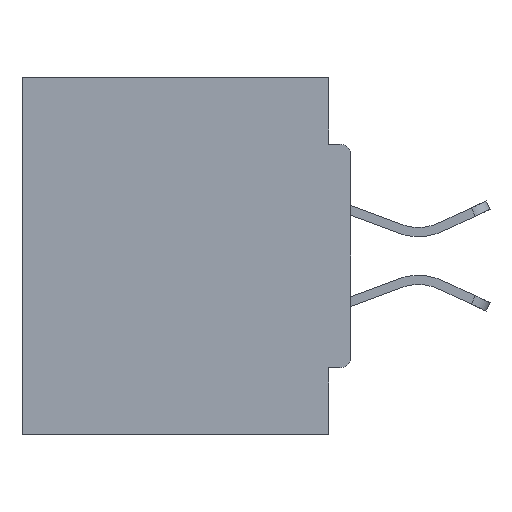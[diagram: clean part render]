
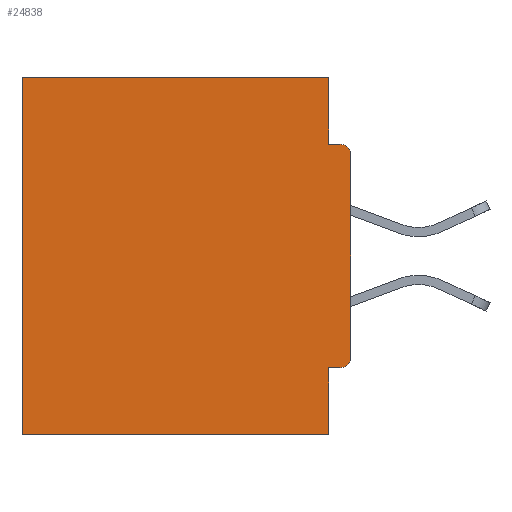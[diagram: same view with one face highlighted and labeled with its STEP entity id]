
A CAD part, left-side view. The second image highlights one B-rep face of the part: STEP entity #24838.
In plain terms, the highlighted planar face has unit normal (-1, 0, 0).
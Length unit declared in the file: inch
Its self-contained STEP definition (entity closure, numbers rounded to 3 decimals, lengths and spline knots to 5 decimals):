
#800 = CARTESIAN_POINT ( 'NONE',  ( 0.298, 0.031, 0. ) ) ;
#1332 = LINE ( 'NONE', #5287, #27914 ) ;
#1962 = LINE ( 'NONE', #23054, #7258 ) ;
#1979 = EDGE_CURVE ( 'NONE', #17527, #6741, #15284, .T. ) ;
#2102 = EDGE_LOOP ( 'NONE', ( #6151, #5456, #30025, #8005, #17587, #11254, #28981, #26179, #26817, #15658 ) ) ;
#2322 = VECTOR ( 'NONE', #16249, 39.37008 ) ;
#2545 = VECTOR ( 'NONE', #28254, 39.37008 ) ;
#3219 = VERTEX_POINT ( 'NONE', #16351 ) ;
#3903 = DIRECTION ( 'NONE',  ( 0., 0., -1. ) ) ;
#4043 = EDGE_CURVE ( 'NONE', #28127, #31841, #24545, .T. ) ;
#4402 = CARTESIAN_POINT ( 'NONE',  ( 0.298, 0., 0. ) ) ;
#5287 = CARTESIAN_POINT ( 'NONE',  ( 0.298, 0., -0.0935 ) ) ;
#5456 = ORIENTED_EDGE ( 'NONE', *, *, #21370, .F. ) ;
#5717 = CARTESIAN_POINT ( 'NONE',  ( 0.298, 0., -0.3915 ) ) ;
#6151 = ORIENTED_EDGE ( 'NONE', *, *, #33785, .T. ) ;
#6346 = AXIS2_PLACEMENT_3D ( 'NONE', #28651, #12652, #20780 ) ;
#6703 = CARTESIAN_POINT ( 'NONE',  ( 0.298, 0.031, -0.5 ) ) ;
#6741 = VERTEX_POINT ( 'NONE', #6703 ) ;
#6881 = DIRECTION ( 'NONE',  ( 0., 0., -1. ) ) ;
#6910 = DIRECTION ( 'NONE',  ( 0., 1., 0. ) ) ;
#7258 = VECTOR ( 'NONE', #28536, 39.37008 ) ;
#7495 = CIRCLE ( 'NONE', #19519, 0.015 ) ;
#7565 = EDGE_CURVE ( 'NONE', #6741, #33610, #25634, .T. ) ;
#8005 = ORIENTED_EDGE ( 'NONE', *, *, #4043, .T. ) ;
#8009 = CARTESIAN_POINT ( 'NONE',  ( 0.298, 0.015, -0.4065 ) ) ;
#9202 = CARTESIAN_POINT ( 'NONE',  ( 0.298, 0.46, 0. ) ) ;
#9961 = CARTESIAN_POINT ( 'NONE',  ( 0.298, 0.031, -0.5 ) ) ;
#9985 = VECTOR ( 'NONE', #30195, 39.37008 ) ;
#10547 = EDGE_CURVE ( 'NONE', #28127, #3219, #14810, .T. ) ;
#10655 = VECTOR ( 'NONE', #6910, 39.37008 ) ;
#11254 = ORIENTED_EDGE ( 'NONE', *, *, #7565, .F. ) ;
#12080 = VERTEX_POINT ( 'NONE', #5717 ) ;
#12652 = DIRECTION ( 'NONE',  ( 1., 0., 0. ) ) ;
#14419 = DIRECTION ( 'NONE',  ( -1., 0., 0. ) ) ;
#14651 = EDGE_CURVE ( 'NONE', #15191, #12080, #16971, .T. ) ;
#14810 = LINE ( 'NONE', #9961, #2545 ) ;
#15191 = VERTEX_POINT ( 'NONE', #8009 ) ;
#15284 = LINE ( 'NONE', #30068, #9985 ) ;
#15658 = ORIENTED_EDGE ( 'NONE', *, *, #26927, .F. ) ;
#16249 = DIRECTION ( 'NONE',  ( 0., 1., 0. ) ) ;
#16351 = CARTESIAN_POINT ( 'NONE',  ( 0.298, 0.031, -0.0935 ) ) ;
#16971 = CIRCLE ( 'NONE', #18334, 0.015 ) ;
#17304 = LINE ( 'NONE', #9202, #26270 ) ;
#17527 = VERTEX_POINT ( 'NONE', #20069 ) ;
#17587 = ORIENTED_EDGE ( 'NONE', *, *, #26203, .T. ) ;
#18246 = DIRECTION ( 'NONE',  ( -1., 0., 0. ) ) ;
#18334 = AXIS2_PLACEMENT_3D ( 'NONE', #30108, #14419, #3903 ) ;
#18360 = DIRECTION ( 'NONE',  ( 0., 0., -1. ) ) ;
#18557 = DIRECTION ( 'NONE',  ( 0., -1., 0. ) ) ;
#19360 = DIRECTION ( 'NONE',  ( 0., 0., -1. ) ) ;
#19519 = AXIS2_PLACEMENT_3D ( 'NONE', #28989, #18246, #18360 ) ;
#20069 = CARTESIAN_POINT ( 'NONE',  ( 0.298, 0.031, -0.4065 ) ) ;
#20092 = CARTESIAN_POINT ( 'NONE',  ( 0.298, 0., -0.1085 ) ) ;
#20466 = CARTESIAN_POINT ( 'NONE',  ( 0.298, 0.46, 0. ) ) ;
#20780 = DIRECTION ( 'NONE',  ( 0., 0., -1. ) ) ;
#21370 = EDGE_CURVE ( 'NONE', #3219, #23972, #1332, .T. ) ;
#22527 = CARTESIAN_POINT ( 'NONE',  ( 0.298, 0.46, -0.5 ) ) ;
#23054 = CARTESIAN_POINT ( 'NONE',  ( 0.298, 0., -0.4065 ) ) ;
#23844 = EDGE_CURVE ( 'NONE', #15191, #17527, #1962, .T. ) ;
#23972 = VERTEX_POINT ( 'NONE', #33205 ) ;
#24545 = LINE ( 'NONE', #4402, #10655 ) ;
#24775 = FACE_OUTER_BOUND ( 'NONE', #2102, .T. ) ;
#24838 = ADVANCED_FACE ( 'NONE', ( #24775 ), #25668, .F. ) ;
#25634 = LINE ( 'NONE', #32250, #2322 ) ;
#25668 = PLANE ( 'NONE',  #6346 ) ;
#26179 = ORIENTED_EDGE ( 'NONE', *, *, #23844, .F. ) ;
#26203 = EDGE_CURVE ( 'NONE', #31841, #33610, #17304, .T. ) ;
#26270 = VECTOR ( 'NONE', #6881, 39.37008 ) ;
#26542 = CARTESIAN_POINT ( 'NONE',  ( 0.298, 0., 0. ) ) ;
#26665 = VERTEX_POINT ( 'NONE', #20092 ) ;
#26817 = ORIENTED_EDGE ( 'NONE', *, *, #14651, .T. ) ;
#26927 = EDGE_CURVE ( 'NONE', #26665, #12080, #32821, .T. ) ;
#27914 = VECTOR ( 'NONE', #18557, 39.37008 ) ;
#28127 = VERTEX_POINT ( 'NONE', #800 ) ;
#28254 = DIRECTION ( 'NONE',  ( 0., 0., -1. ) ) ;
#28536 = DIRECTION ( 'NONE',  ( 0., 1., 0. ) ) ;
#28651 = CARTESIAN_POINT ( 'NONE',  ( 0.298, 0., 0. ) ) ;
#28981 = ORIENTED_EDGE ( 'NONE', *, *, #1979, .F. ) ;
#28989 = CARTESIAN_POINT ( 'NONE',  ( 0.298, 0.015, -0.1085 ) ) ;
#30025 = ORIENTED_EDGE ( 'NONE', *, *, #10547, .F. ) ;
#30068 = CARTESIAN_POINT ( 'NONE',  ( 0.298, 0.031, -0.5 ) ) ;
#30108 = CARTESIAN_POINT ( 'NONE',  ( 0.298, 0.015, -0.3915 ) ) ;
#30195 = DIRECTION ( 'NONE',  ( 0., 0., -1. ) ) ;
#30792 = VECTOR ( 'NONE', #19360, 39.37008 ) ;
#31841 = VERTEX_POINT ( 'NONE', #20466 ) ;
#32250 = CARTESIAN_POINT ( 'NONE',  ( 0.298, 0., -0.5 ) ) ;
#32821 = LINE ( 'NONE', #26542, #30792 ) ;
#33205 = CARTESIAN_POINT ( 'NONE',  ( 0.298, 0.015, -0.0935 ) ) ;
#33610 = VERTEX_POINT ( 'NONE', #22527 ) ;
#33785 = EDGE_CURVE ( 'NONE', #26665, #23972, #7495, .T. ) ;
